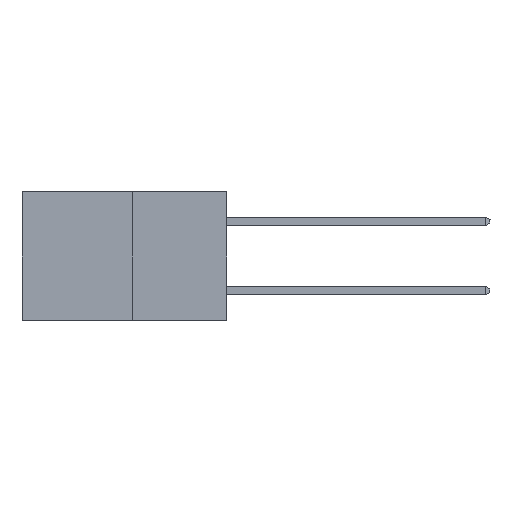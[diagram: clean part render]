
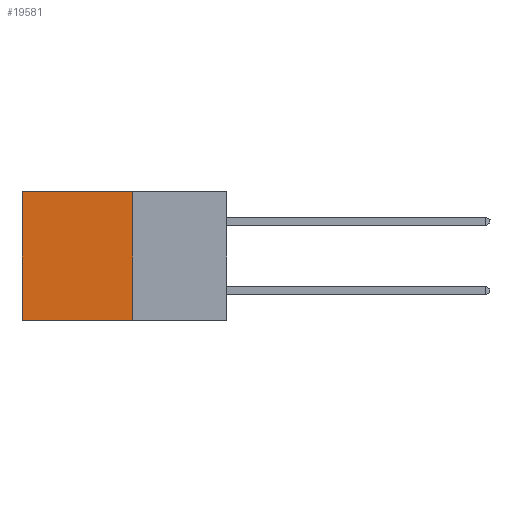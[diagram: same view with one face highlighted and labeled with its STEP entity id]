
A CAD part, left-side view. The second image highlights one B-rep face of the part: STEP entity #19581.
In plain terms, the highlighted planar face has unit normal (-1, 0, 0).
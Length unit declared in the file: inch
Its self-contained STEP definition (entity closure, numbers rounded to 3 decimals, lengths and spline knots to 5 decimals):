
#369 = CARTESIAN_POINT ( 'NONE',  ( 0.277, 0.27, -0.37 ) ) ;
#836 = LINE ( 'NONE', #20484, #12740 ) ;
#962 = CARTESIAN_POINT ( 'NONE',  ( 0.277, 0.59, -0.37 ) ) ;
#3075 = EDGE_CURVE ( 'NONE', #4634, #11752, #6630, .T. ) ;
#3355 = EDGE_CURVE ( 'NONE', #14171, #4634, #836, .T. ) ;
#4634 = VERTEX_POINT ( 'NONE', #4860 ) ;
#4860 = CARTESIAN_POINT ( 'NONE',  ( 0.277, 0.59, 0. ) ) ;
#4890 = DIRECTION ( 'NONE',  ( 0., 0., -1. ) ) ;
#5144 = VERTEX_POINT ( 'NONE', #11789 ) ;
#5592 = CARTESIAN_POINT ( 'NONE',  ( 0.277, 0.27, -0.37 ) ) ;
#5894 = LINE ( 'NONE', #369, #13279 ) ;
#6630 = LINE ( 'NONE', #16015, #7144 ) ;
#6860 = EDGE_CURVE ( 'NONE', #14171, #5144, #17041, .T. ) ;
#7144 = VECTOR ( 'NONE', #19893, 39.37008 ) ;
#8482 = CARTESIAN_POINT ( 'NONE',  ( 0.277, 0.27, -0.37 ) ) ;
#8572 = EDGE_LOOP ( 'NONE', ( #16112, #17143, #17653, #18150 ) ) ;
#10347 = PLANE ( 'NONE',  #17321 ) ;
#10420 = DIRECTION ( 'NONE',  ( 0., 0., -1. ) ) ;
#11752 = VERTEX_POINT ( 'NONE', #962 ) ;
#11789 = CARTESIAN_POINT ( 'NONE',  ( 0.277, 0.27, -0.37 ) ) ;
#12740 = VECTOR ( 'NONE', #20631, 39.37008 ) ;
#13279 = VECTOR ( 'NONE', #16471, 39.37008 ) ;
#14171 = VERTEX_POINT ( 'NONE', #19672 ) ;
#16015 = CARTESIAN_POINT ( 'NONE',  ( 0.277, 0.59, -0.37 ) ) ;
#16112 = ORIENTED_EDGE ( 'NONE', *, *, #3075, .T. ) ;
#16471 = DIRECTION ( 'NONE',  ( 0., 1., 0. ) ) ;
#16522 = VECTOR ( 'NONE', #4890, 39.37008 ) ;
#17041 = LINE ( 'NONE', #8482, #16522 ) ;
#17143 = ORIENTED_EDGE ( 'NONE', *, *, #19543, .F. ) ;
#17321 = AXIS2_PLACEMENT_3D ( 'NONE', #5592, #19860, #10420 ) ;
#17653 = ORIENTED_EDGE ( 'NONE', *, *, #6860, .F. ) ;
#18150 = ORIENTED_EDGE ( 'NONE', *, *, #3355, .T. ) ;
#19543 = EDGE_CURVE ( 'NONE', #5144, #11752, #5894, .T. ) ;
#19581 = ADVANCED_FACE ( 'NONE', ( #20792 ), #10347, .F. ) ;
#19672 = CARTESIAN_POINT ( 'NONE',  ( 0.277, 0.27, 0. ) ) ;
#19860 = DIRECTION ( 'NONE',  ( 1., 0., 0. ) ) ;
#19893 = DIRECTION ( 'NONE',  ( 0., 0., -1. ) ) ;
#20484 = CARTESIAN_POINT ( 'NONE',  ( 0.277, 0.27, 0. ) ) ;
#20631 = DIRECTION ( 'NONE',  ( 0., 1., 0. ) ) ;
#20792 = FACE_OUTER_BOUND ( 'NONE', #8572, .T. ) ;
